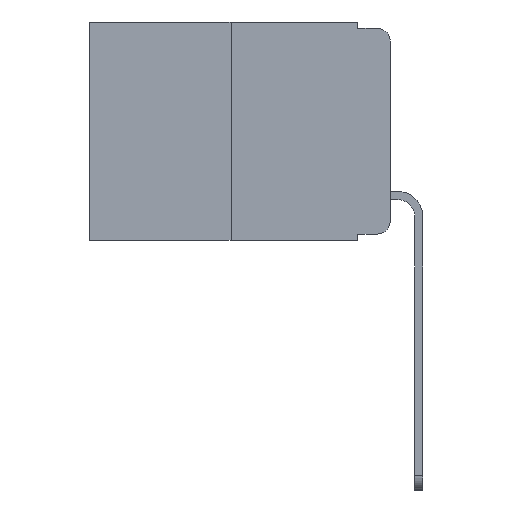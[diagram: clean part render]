
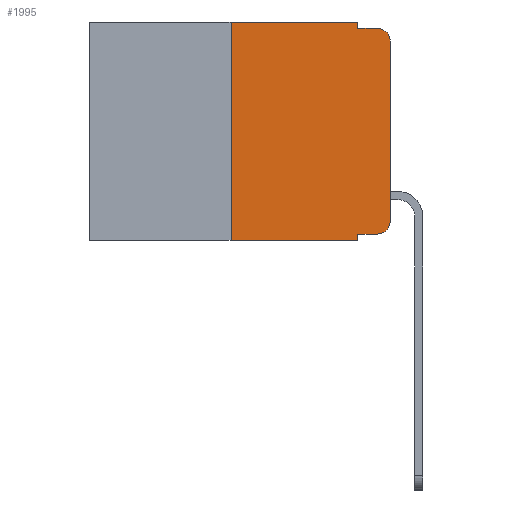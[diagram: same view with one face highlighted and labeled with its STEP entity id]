
A CAD part, left-side view. The second image highlights one B-rep face of the part: STEP entity #1995.
In plain terms, the highlighted planar face has unit normal (-1, 0, 0).
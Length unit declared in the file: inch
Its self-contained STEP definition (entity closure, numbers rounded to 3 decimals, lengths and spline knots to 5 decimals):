
#369 = EDGE_CURVE ( 'NONE', #7515, #6372, #7636, .T. ) ;
#439 = ORIENTED_EDGE ( 'NONE', *, *, #4900, .T. ) ;
#491 = VERTEX_POINT ( 'NONE', #12298 ) ;
#627 = CARTESIAN_POINT ( 'NONE',  ( 0., 0.02, -0.333 ) ) ;
#852 = LINE ( 'NONE', #8710, #10758 ) ;
#904 = EDGE_CURVE ( 'NONE', #6523, #5354, #11642, .T. ) ;
#909 = VERTEX_POINT ( 'NONE', #1933 ) ;
#914 = DIRECTION ( 'NONE',  ( 0., 0., -1. ) ) ;
#936 = CARTESIAN_POINT ( 'NONE',  ( 0., 0.051, 0. ) ) ;
#1130 = VECTOR ( 'NONE', #6096, 39.37008 ) ;
#1143 = DIRECTION ( 'NONE',  ( -1., 0., 0. ) ) ;
#1152 = CARTESIAN_POINT ( 'NONE',  ( 0., 0.051, -0.333 ) ) ;
#1358 = VECTOR ( 'NONE', #7588, 39.37008 ) ;
#1902 = ORIENTED_EDGE ( 'NONE', *, *, #6955, .F. ) ;
#1933 = CARTESIAN_POINT ( 'NONE',  ( 0., 0., -0.313 ) ) ;
#1971 = DIRECTION ( 'NONE',  ( 0., 0., -1. ) ) ;
#1995 = ADVANCED_FACE ( 'NONE', ( #9921 ), #10763, .F. ) ;
#2010 = LINE ( 'NONE', #5680, #9352 ) ;
#2153 = DIRECTION ( 'NONE',  ( 0., -1., 0. ) ) ;
#2160 = CARTESIAN_POINT ( 'NONE',  ( 0., 0.473, 0. ) ) ;
#2296 = EDGE_CURVE ( 'NONE', #7592, #909, #6698, .T. ) ;
#2493 = CARTESIAN_POINT ( 'NONE',  ( 0., 0.473, -0.343 ) ) ;
#2703 = ORIENTED_EDGE ( 'NONE', *, *, #904, .F. ) ;
#3430 = ORIENTED_EDGE ( 'NONE', *, *, #10860, .F. ) ;
#3557 = VERTEX_POINT ( 'NONE', #11119 ) ;
#3718 = EDGE_LOOP ( 'NONE', ( #8640, #439, #1902, #3430, #2703, #11362, #4345, #8774, #6594, #7304 ) ) ;
#3807 = CARTESIAN_POINT ( 'NONE',  ( 0., 0.051, 0. ) ) ;
#4047 = LINE ( 'NONE', #11237, #1358 ) ;
#4098 = VERTEX_POINT ( 'NONE', #11903 ) ;
#4204 = DIRECTION ( 'NONE',  ( 0., 0., -1. ) ) ;
#4345 = ORIENTED_EDGE ( 'NONE', *, *, #369, .T. ) ;
#4828 = LINE ( 'NONE', #10554, #9795 ) ;
#4880 = CARTESIAN_POINT ( 'NONE',  ( 0., 0.02, -0.03 ) ) ;
#4900 = EDGE_CURVE ( 'NONE', #4098, #6025, #7627, .T. ) ;
#4944 = EDGE_CURVE ( 'NONE', #491, #6372, #4828, .T. ) ;
#5173 = CARTESIAN_POINT ( 'NONE',  ( 0., 0.25, 0. ) ) ;
#5255 = DIRECTION ( 'NONE',  ( 0., 0., -1. ) ) ;
#5354 = VERTEX_POINT ( 'NONE', #3807 ) ;
#5437 = VECTOR ( 'NONE', #11009, 39.37008 ) ;
#5680 = CARTESIAN_POINT ( 'NONE',  ( 0., 0., 0. ) ) ;
#6025 = VERTEX_POINT ( 'NONE', #9169 ) ;
#6096 = DIRECTION ( 'NONE',  ( 0., -1., 0. ) ) ;
#6354 = AXIS2_PLACEMENT_3D ( 'NONE', #8926, #7757, #5255 ) ;
#6372 = VERTEX_POINT ( 'NONE', #6836 ) ;
#6523 = VERTEX_POINT ( 'NONE', #5173 ) ;
#6594 = ORIENTED_EDGE ( 'NONE', *, *, #9661, .T. ) ;
#6630 = LINE ( 'NONE', #1152, #1130 ) ;
#6698 = CIRCLE ( 'NONE', #6354, 0.02 ) ;
#6836 = CARTESIAN_POINT ( 'NONE',  ( 0., 0.051, -0.343 ) ) ;
#6955 = EDGE_CURVE ( 'NONE', #3557, #6025, #4047, .T. ) ;
#6995 = AXIS2_PLACEMENT_3D ( 'NONE', #4880, #1143, #4204 ) ;
#7157 = VECTOR ( 'NONE', #1971, 39.37008 ) ;
#7304 = ORIENTED_EDGE ( 'NONE', *, *, #2296, .T. ) ;
#7366 = CARTESIAN_POINT ( 'NONE',  ( 0., 0.25, -0.343 ) ) ;
#7515 = VERTEX_POINT ( 'NONE', #7366 ) ;
#7588 = DIRECTION ( 'NONE',  ( 0., -1., 0. ) ) ;
#7592 = VERTEX_POINT ( 'NONE', #627 ) ;
#7627 = CIRCLE ( 'NONE', #6995, 0.02 ) ;
#7636 = LINE ( 'NONE', #2493, #5437 ) ;
#7757 = DIRECTION ( 'NONE',  ( -1., 0., 0. ) ) ;
#8520 = DIRECTION ( 'NONE',  ( 0., 0., 1. ) ) ;
#8640 = ORIENTED_EDGE ( 'NONE', *, *, #11361, .T. ) ;
#8710 = CARTESIAN_POINT ( 'NONE',  ( 0., 0.25, 0. ) ) ;
#8774 = ORIENTED_EDGE ( 'NONE', *, *, #4944, .F. ) ;
#8926 = CARTESIAN_POINT ( 'NONE',  ( 0., 0.02, -0.313 ) ) ;
#9169 = CARTESIAN_POINT ( 'NONE',  ( 0., 0.02, -0.01 ) ) ;
#9352 = VECTOR ( 'NONE', #8520, 39.37008 ) ;
#9382 = CARTESIAN_POINT ( 'NONE',  ( 0., 0.473, 0. ) ) ;
#9634 = DIRECTION ( 'NONE',  ( 0., 0., 1. ) ) ;
#9661 = EDGE_CURVE ( 'NONE', #491, #7592, #6630, .T. ) ;
#9795 = VECTOR ( 'NONE', #914, 39.37008 ) ;
#9921 = FACE_OUTER_BOUND ( 'NONE', #3718, .T. ) ;
#9936 = LINE ( 'NONE', #936, #7157 ) ;
#10554 = CARTESIAN_POINT ( 'NONE',  ( 0., 0.051, 0. ) ) ;
#10758 = VECTOR ( 'NONE', #9634, 39.37008 ) ;
#10763 = PLANE ( 'NONE',  #11769 ) ;
#10764 = DIRECTION ( 'NONE',  ( 0., 0., -1. ) ) ;
#10860 = EDGE_CURVE ( 'NONE', #5354, #3557, #9936, .T. ) ;
#11009 = DIRECTION ( 'NONE',  ( 0., -1., 0. ) ) ;
#11119 = CARTESIAN_POINT ( 'NONE',  ( 0., 0.051, -0.01 ) ) ;
#11237 = CARTESIAN_POINT ( 'NONE',  ( 0., 0.051, -0.01 ) ) ;
#11349 = VECTOR ( 'NONE', #2153, 39.37008 ) ;
#11361 = EDGE_CURVE ( 'NONE', #909, #4098, #2010, .T. ) ;
#11362 = ORIENTED_EDGE ( 'NONE', *, *, #12146, .F. ) ;
#11642 = LINE ( 'NONE', #2160, #11349 ) ;
#11769 = AXIS2_PLACEMENT_3D ( 'NONE', #9382, #11867, #10764 ) ;
#11867 = DIRECTION ( 'NONE',  ( 1., 0., 0. ) ) ;
#11903 = CARTESIAN_POINT ( 'NONE',  ( 0., 0., -0.03 ) ) ;
#12146 = EDGE_CURVE ( 'NONE', #7515, #6523, #852, .T. ) ;
#12298 = CARTESIAN_POINT ( 'NONE',  ( 0., 0.051, -0.333 ) ) ;
